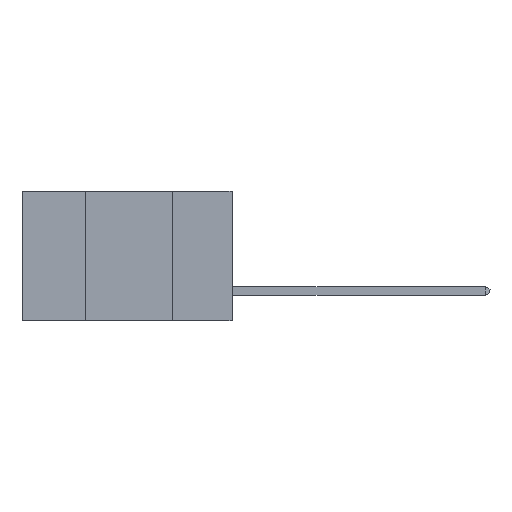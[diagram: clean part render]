
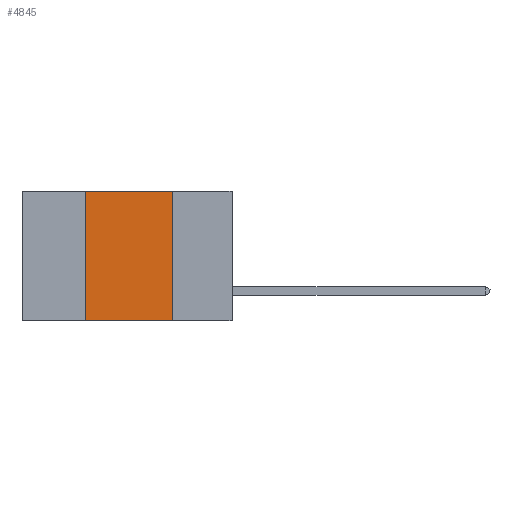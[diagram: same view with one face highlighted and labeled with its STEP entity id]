
A CAD part, left-side view. The second image highlights one B-rep face of the part: STEP entity #4845.
In plain terms, the highlighted planar face has unit normal (-1, 0, 0).
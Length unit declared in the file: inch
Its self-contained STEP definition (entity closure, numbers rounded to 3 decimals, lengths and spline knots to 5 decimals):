
#255 = VERTEX_POINT ( 'NONE', #676 ) ;
#331 = VECTOR ( 'NONE', #5445, 39.37008 ) ;
#471 = LINE ( 'NONE', #3410, #331 ) ;
#676 = CARTESIAN_POINT ( 'NONE',  ( 0., 0.42, 0. ) ) ;
#952 = CARTESIAN_POINT ( 'NONE',  ( 0., 0.6, -0.37 ) ) ;
#1469 = CARTESIAN_POINT ( 'NONE',  ( 0., 0.17, 0. ) ) ;
#1768 = DIRECTION ( 'NONE',  ( 1., 0., 0. ) ) ;
#2179 = ORIENTED_EDGE ( 'NONE', *, *, #7194, .F. ) ;
#2785 = FACE_OUTER_BOUND ( 'NONE', #10276, .T. ) ;
#3319 = CARTESIAN_POINT ( 'NONE',  ( 0., 0.17, 0. ) ) ;
#3410 = CARTESIAN_POINT ( 'NONE',  ( 0., 0.42, 0. ) ) ;
#3823 = ORIENTED_EDGE ( 'NONE', *, *, #6718, .F. ) ;
#4797 = LINE ( 'NONE', #952, #6059 ) ;
#4845 = ADVANCED_FACE ( 'NONE', ( #2785 ), #6149, .F. ) ;
#5295 = CARTESIAN_POINT ( 'NONE',  ( 0., 0.6, 0. ) ) ;
#5348 = VERTEX_POINT ( 'NONE', #6014 ) ;
#5445 = DIRECTION ( 'NONE',  ( 0., 0., 1. ) ) ;
#5508 = VECTOR ( 'NONE', #11141, 39.37008 ) ;
#5697 = VERTEX_POINT ( 'NONE', #6934 ) ;
#6014 = CARTESIAN_POINT ( 'NONE',  ( 0., 0.17, -0.37 ) ) ;
#6059 = VECTOR ( 'NONE', #8986, 39.37008 ) ;
#6092 = DIRECTION ( 'NONE',  ( 0., -1., 0. ) ) ;
#6149 = PLANE ( 'NONE',  #6566 ) ;
#6566 = AXIS2_PLACEMENT_3D ( 'NONE', #7082, #1768, #10588 ) ;
#6718 = EDGE_CURVE ( 'NONE', #8628, #5348, #10161, .T. ) ;
#6934 = CARTESIAN_POINT ( 'NONE',  ( 0., 0.42, -0.37 ) ) ;
#7082 = CARTESIAN_POINT ( 'NONE',  ( 0., 0.6, 0. ) ) ;
#7175 = ORIENTED_EDGE ( 'NONE', *, *, #9493, .F. ) ;
#7194 = EDGE_CURVE ( 'NONE', #255, #8628, #9865, .T. ) ;
#7362 = EDGE_CURVE ( 'NONE', #5697, #5348, #4797, .T. ) ;
#8628 = VERTEX_POINT ( 'NONE', #1469 ) ;
#8925 = VECTOR ( 'NONE', #6092, 39.37008 ) ;
#8986 = DIRECTION ( 'NONE',  ( 0., -1., 0. ) ) ;
#9075 = ORIENTED_EDGE ( 'NONE', *, *, #7362, .T. ) ;
#9493 = EDGE_CURVE ( 'NONE', #5697, #255, #471, .T. ) ;
#9865 = LINE ( 'NONE', #5295, #8925 ) ;
#10161 = LINE ( 'NONE', #3319, #5508 ) ;
#10276 = EDGE_LOOP ( 'NONE', ( #3823, #2179, #7175, #9075 ) ) ;
#10588 = DIRECTION ( 'NONE',  ( 0., 0., -1. ) ) ;
#11141 = DIRECTION ( 'NONE',  ( 0., 0., -1. ) ) ;
